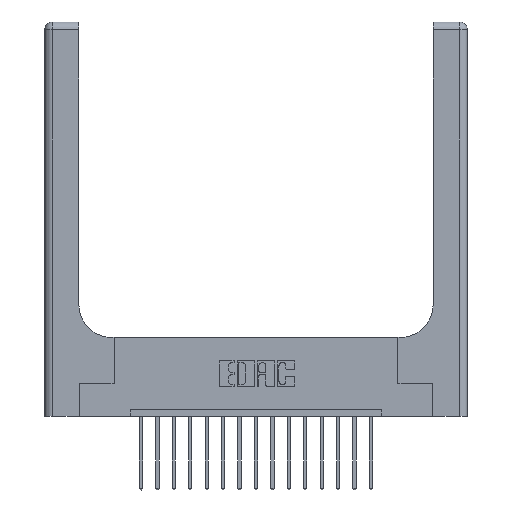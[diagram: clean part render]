
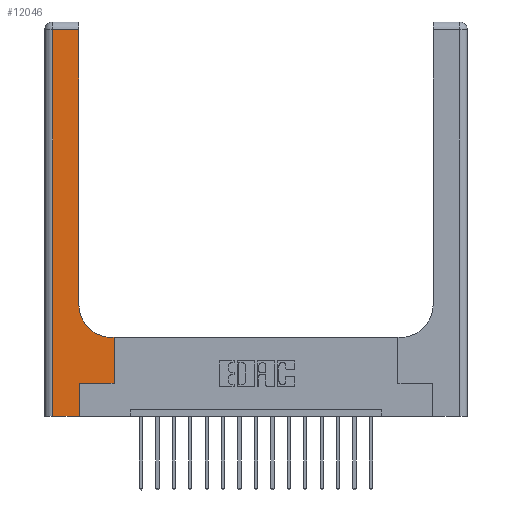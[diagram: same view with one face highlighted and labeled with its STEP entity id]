
A CAD part, top view. The second image highlights one B-rep face of the part: STEP entity #12046.
In plain terms, the highlighted planar face has unit normal (0, 0, 1).
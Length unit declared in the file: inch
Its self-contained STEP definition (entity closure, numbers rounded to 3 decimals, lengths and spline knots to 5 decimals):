
#307 = LINE ( 'NONE', #8234, #2298 ) ;
#361 = CARTESIAN_POINT ( 'NONE',  ( 0.26, 0.6, 0.37 ) ) ;
#495 = CARTESIAN_POINT ( 'NONE',  ( 0.265, 0., 0.37 ) ) ;
#689 = VECTOR ( 'NONE', #5366, 39.37008 ) ;
#700 = AXIS2_PLACEMENT_3D ( 'NONE', #4201, #5569, #11217 ) ;
#908 = LINE ( 'NONE', #12358, #689 ) ;
#1556 = VERTEX_POINT ( 'NONE', #11442 ) ;
#2273 = EDGE_CURVE ( 'NONE', #17362, #14568, #307, .T. ) ;
#2298 = VECTOR ( 'NONE', #8719, 39.37008 ) ;
#2343 = EDGE_LOOP ( 'NONE', ( #11437, #2400, #12251, #10186, #15022, #5417, #7757, #6903, #11786 ) ) ;
#2396 = VECTOR ( 'NONE', #7604, 39.37008 ) ;
#2400 = ORIENTED_EDGE ( 'NONE', *, *, #2273, .T. ) ;
#2724 = AXIS2_PLACEMENT_3D ( 'NONE', #4422, #3082, #12818 ) ;
#3034 = VERTEX_POINT ( 'NONE', #495 ) ;
#3082 = DIRECTION ( 'NONE',  ( 0., 0., -1. ) ) ;
#3476 = VERTEX_POINT ( 'NONE', #12477 ) ;
#3811 = VERTEX_POINT ( 'NONE', #10546 ) ;
#4201 = CARTESIAN_POINT ( 'NONE',  ( 0.51, 0.85, 0.37 ) ) ;
#4422 = CARTESIAN_POINT ( 'NONE',  ( 0., 3., 0.37 ) ) ;
#4478 = PLANE ( 'NONE',  #2724 ) ;
#4509 = EDGE_CURVE ( 'NONE', #5675, #1556, #8774, .T. ) ;
#4694 = CARTESIAN_POINT ( 'NONE',  ( 0.26, 0.85, 0.37 ) ) ;
#4738 = EDGE_CURVE ( 'NONE', #5068, #17362, #10730, .T. ) ;
#5068 = VERTEX_POINT ( 'NONE', #4694 ) ;
#5366 = DIRECTION ( 'NONE',  ( 0., 1., 0. ) ) ;
#5417 = ORIENTED_EDGE ( 'NONE', *, *, #4509, .T. ) ;
#5511 = LINE ( 'NONE', #15883, #9697 ) ;
#5566 = EDGE_CURVE ( 'NONE', #3476, #3811, #15294, .T. ) ;
#5569 = DIRECTION ( 'NONE',  ( 0., 0., -1. ) ) ;
#5675 = VERTEX_POINT ( 'NONE', #13083 ) ;
#6174 = CIRCLE ( 'NONE', #700, 0.25 ) ;
#6903 = ORIENTED_EDGE ( 'NONE', *, *, #5566, .T. ) ;
#7480 = LINE ( 'NONE', #8837, #15598 ) ;
#7604 = DIRECTION ( 'NONE',  ( 1., 0., 0. ) ) ;
#7757 = ORIENTED_EDGE ( 'NONE', *, *, #8180, .T. ) ;
#8180 = EDGE_CURVE ( 'NONE', #1556, #3476, #908, .T. ) ;
#8196 = CARTESIAN_POINT ( 'NONE',  ( 0.06, 0., 0.37 ) ) ;
#8234 = CARTESIAN_POINT ( 'NONE',  ( 0., 2.94, 0.37 ) ) ;
#8691 = DIRECTION ( 'NONE',  ( -1., 0., 0. ) ) ;
#8719 = DIRECTION ( 'NONE',  ( -1., 0., 0. ) ) ;
#8774 = LINE ( 'NONE', #13070, #2396 ) ;
#8837 = CARTESIAN_POINT ( 'NONE',  ( 0., 0., 0.37 ) ) ;
#9114 = EDGE_CURVE ( 'NONE', #3034, #5675, #15154, .T. ) ;
#9164 = VECTOR ( 'NONE', #8691, 39.37008 ) ;
#9697 = VECTOR ( 'NONE', #13301, 39.37008 ) ;
#9875 = VECTOR ( 'NONE', #17971, 39.37008 ) ;
#10186 = ORIENTED_EDGE ( 'NONE', *, *, #13730, .T. ) ;
#10546 = CARTESIAN_POINT ( 'NONE',  ( 0.51, 0.6, 0.37 ) ) ;
#10730 = LINE ( 'NONE', #17796, #9875 ) ;
#11217 = DIRECTION ( 'NONE',  ( 1., 0., 0. ) ) ;
#11437 = ORIENTED_EDGE ( 'NONE', *, *, #4738, .T. ) ;
#11442 = CARTESIAN_POINT ( 'NONE',  ( 0.528, 0.25, 0.37 ) ) ;
#11475 = DIRECTION ( 'NONE',  ( 1., 0., 0. ) ) ;
#11786 = ORIENTED_EDGE ( 'NONE', *, *, #13410, .T. ) ;
#12046 = ADVANCED_FACE ( 'NONE', ( #14090 ), #4478, .F. ) ;
#12251 = ORIENTED_EDGE ( 'NONE', *, *, #18116, .T. ) ;
#12358 = CARTESIAN_POINT ( 'NONE',  ( 0.528, 0.25, 0.37 ) ) ;
#12477 = CARTESIAN_POINT ( 'NONE',  ( 0.528, 0.6, 0.37 ) ) ;
#12818 = DIRECTION ( 'NONE',  ( -1., 0., 0. ) ) ;
#13070 = CARTESIAN_POINT ( 'NONE',  ( 0.265, 0.25, 0.37 ) ) ;
#13083 = CARTESIAN_POINT ( 'NONE',  ( 0.265, 0.25, 0.37 ) ) ;
#13301 = DIRECTION ( 'NONE',  ( 0., -1., 0. ) ) ;
#13341 = CARTESIAN_POINT ( 'NONE',  ( 0.06, 2.94, 0.37 ) ) ;
#13403 = VECTOR ( 'NONE', #15067, 39.37008 ) ;
#13410 = EDGE_CURVE ( 'NONE', #3811, #5068, #6174, .T. ) ;
#13627 = CARTESIAN_POINT ( 'NONE',  ( 0.26, 2.94, 0.37 ) ) ;
#13730 = EDGE_CURVE ( 'NONE', #15857, #3034, #7480, .T. ) ;
#14090 = FACE_OUTER_BOUND ( 'NONE', #2343, .T. ) ;
#14568 = VERTEX_POINT ( 'NONE', #13341 ) ;
#15022 = ORIENTED_EDGE ( 'NONE', *, *, #9114, .T. ) ;
#15067 = DIRECTION ( 'NONE',  ( 0., 1., 0. ) ) ;
#15154 = LINE ( 'NONE', #16352, #13403 ) ;
#15294 = LINE ( 'NONE', #361, #9164 ) ;
#15598 = VECTOR ( 'NONE', #11475, 39.37008 ) ;
#15857 = VERTEX_POINT ( 'NONE', #8196 ) ;
#15883 = CARTESIAN_POINT ( 'NONE',  ( 0.06, 3., 0.37 ) ) ;
#16352 = CARTESIAN_POINT ( 'NONE',  ( 0.265, 0., 0.37 ) ) ;
#17362 = VERTEX_POINT ( 'NONE', #13627 ) ;
#17796 = CARTESIAN_POINT ( 'NONE',  ( 0.26, 3., 0.37 ) ) ;
#17971 = DIRECTION ( 'NONE',  ( 0., 1., 0. ) ) ;
#18116 = EDGE_CURVE ( 'NONE', #14568, #15857, #5511, .T. ) ;
